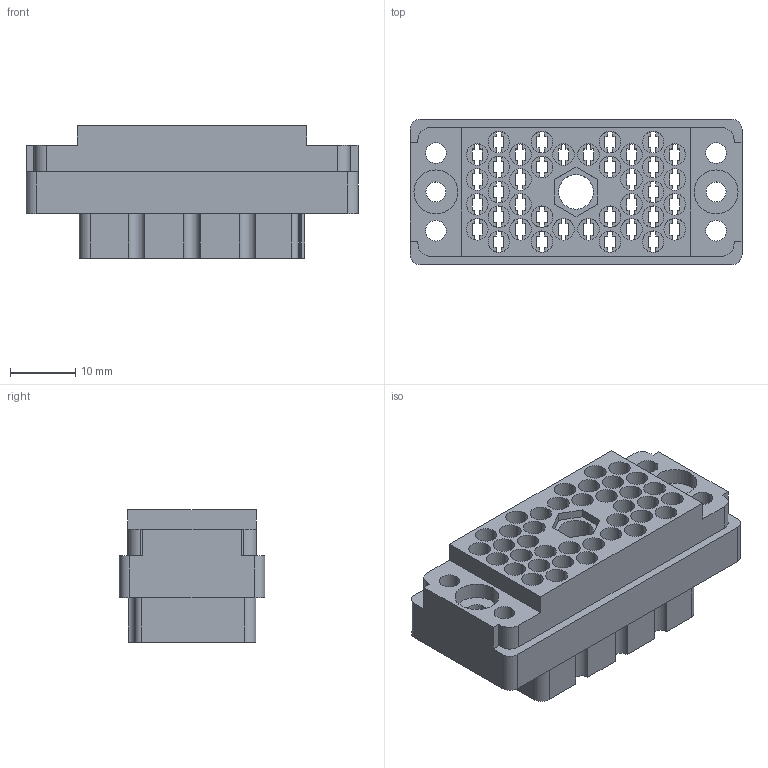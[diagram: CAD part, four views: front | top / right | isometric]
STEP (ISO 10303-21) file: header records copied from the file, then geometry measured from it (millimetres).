
FILE_DESCRIPTION (( 'STEP AP203' ), '1' );
FILE_NAME ('516-038-000-400.STEP', '2020-03-04T21:41:24', ( '' ), ( '' ), 'SwSTEP 2.0', 'SolidWorks 2016', '' );
FILE_SCHEMA (( 'CONFIG_CONTROL_DESIGN' ));
Length unit declared in the file: inch
Products named in the file (2): 516-038-000-400; 516 Part Receptacle_038
Assembly tree (1 placements, depth 2):
  516-038-000-400
    516 Part Receptacle_038
Bounding box: 50.8 x 22.25 x 20.27 mm (x, y, z)
Volume: 10578.9 mm3; surface area: 14493.4 mm2
Topology: 1 solids, 1 shells, 917 faces, 2696 edges, 1796 vertices
Faces by surface type: plane 637, cylinder 278, cone 2
Entity records: 30927 total; most frequent: CARTESIAN_POINT 5413, ORIENTED_EDGE 5392, DIRECTION 5247, EDGE_CURVE 2696, LINE 1987, VECTOR 1987, VERTEX_POINT 1796, AXIS2_PLACEMENT_3D 1630
